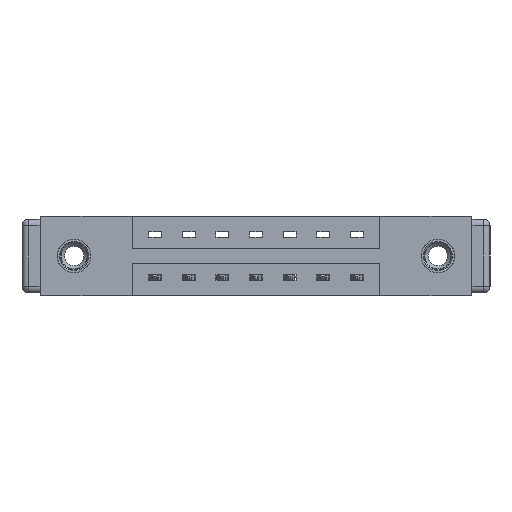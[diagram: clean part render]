
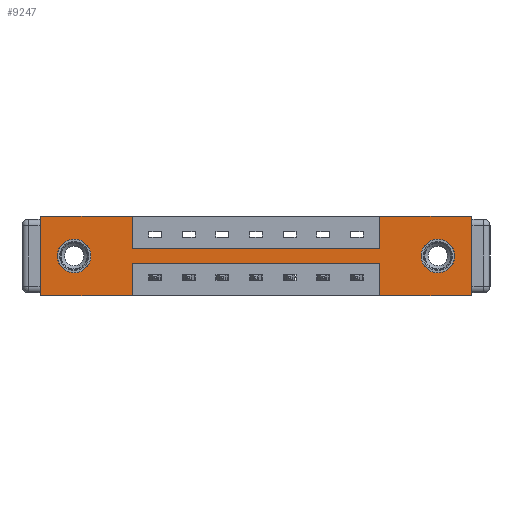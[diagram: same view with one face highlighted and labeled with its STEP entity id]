
A CAD part, front view. The second image highlights one B-rep face of the part: STEP entity #9247.
In plain terms, the highlighted planar face has unit normal (0, -1, 0).
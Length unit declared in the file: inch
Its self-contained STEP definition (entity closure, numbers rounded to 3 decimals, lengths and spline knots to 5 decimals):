
#41 = LINE ( 'NONE', #3227, #10011 ) ;
#83 = EDGE_CURVE ( 'NONE', #3918, #10486, #2257, .T. ) ;
#154 = DIRECTION ( 'NONE',  ( 0., 0., -1. ) ) ;
#155 = EDGE_CURVE ( 'NONE', #5414, #1514, #12267, .T. ) ;
#390 = LINE ( 'NONE', #3840, #11283 ) ;
#429 = AXIS2_PLACEMENT_3D ( 'NONE', #11766, #8809, #8047 ) ;
#773 = VECTOR ( 'NONE', #5761, 39.37008 ) ;
#810 = ORIENTED_EDGE ( 'NONE', *, *, #155, .T. ) ;
#975 = DIRECTION ( 'NONE',  ( 0., 0., 1. ) ) ;
#1060 = CARTESIAN_POINT ( 'NONE',  ( 0.425, 0., -0.22 ) ) ;
#1147 = VECTOR ( 'NONE', #5138, 39.37008 ) ;
#1182 = ORIENTED_EDGE ( 'NONE', *, *, #2270, .T. ) ;
#1375 = LINE ( 'NONE', #10587, #773 ) ;
#1454 = EDGE_CURVE ( 'NONE', #12135, #6594, #2813, .T. ) ;
#1498 = CARTESIAN_POINT ( 'NONE',  ( 0.155, 0., -0.263 ) ) ;
#1514 = VERTEX_POINT ( 'NONE', #2325 ) ;
#1581 = DIRECTION ( 'NONE',  ( 1., 0., 0. ) ) ;
#1786 = VECTOR ( 'NONE', #6313, 39.37008 ) ;
#1788 = CARTESIAN_POINT ( 'NONE',  ( 0.425, 0., -0.37 ) ) ;
#1835 = DIRECTION ( 'NONE',  ( 1., 0., 0. ) ) ;
#1883 = LINE ( 'NONE', #5385, #12038 ) ;
#1897 = VERTEX_POINT ( 'NONE', #5158 ) ;
#2151 = CARTESIAN_POINT ( 'NONE',  ( 0.155, 0., -0.185 ) ) ;
#2257 = LINE ( 'NONE', #3065, #8626 ) ;
#2270 = EDGE_CURVE ( 'NONE', #9743, #3551, #11483, .T. ) ;
#2309 = EDGE_CURVE ( 'NONE', #3551, #9743, #4194, .T. ) ;
#2325 = CARTESIAN_POINT ( 'NONE',  ( 1.843, 0., -0.263 ) ) ;
#2339 = EDGE_LOOP ( 'NONE', ( #3358, #3071, #7086, #3645, #11951, #3665, #6571, #7461, #10893, #12211, #9623, #10466 ) ) ;
#2487 = DIRECTION ( 'NONE',  ( 0., 1., 0. ) ) ;
#2681 = AXIS2_PLACEMENT_3D ( 'NONE', #10922, #7076, #11890 ) ;
#2778 = DIRECTION ( 'NONE',  ( 0., 0., -1. ) ) ;
#2813 = LINE ( 'NONE', #11980, #1786 ) ;
#2863 = CARTESIAN_POINT ( 'NONE',  ( 0., 0., 0. ) ) ;
#2952 = EDGE_CURVE ( 'NONE', #7847, #11902, #11616, .T. ) ;
#3065 = CARTESIAN_POINT ( 'NONE',  ( 0., 0., 0. ) ) ;
#3071 = ORIENTED_EDGE ( 'NONE', *, *, #2952, .F. ) ;
#3073 = DIRECTION ( 'NONE',  ( -1., 0., 0. ) ) ;
#3104 = DIRECTION ( 'NONE',  ( -1., 0., 0. ) ) ;
#3227 = CARTESIAN_POINT ( 'NONE',  ( 1.573, 0., -0.37 ) ) ;
#3345 = AXIS2_PLACEMENT_3D ( 'NONE', #2151, #4499, #4542 ) ;
#3358 = ORIENTED_EDGE ( 'NONE', *, *, #10921, .F. ) ;
#3420 = VERTEX_POINT ( 'NONE', #6747 ) ;
#3512 = LINE ( 'NONE', #2863, #6861 ) ;
#3551 = VERTEX_POINT ( 'NONE', #1498 ) ;
#3641 = LINE ( 'NONE', #1788, #9851 ) ;
#3645 = ORIENTED_EDGE ( 'NONE', *, *, #10880, .F. ) ;
#3658 = CIRCLE ( 'NONE', #6306, 0.078 ) ;
#3665 = ORIENTED_EDGE ( 'NONE', *, *, #9905, .F. ) ;
#3703 = EDGE_CURVE ( 'NONE', #11402, #1897, #1883, .T. ) ;
#3739 = DIRECTION ( 'NONE',  ( 1., 0., 0. ) ) ;
#3840 = CARTESIAN_POINT ( 'NONE',  ( 0., 0., -0.37 ) ) ;
#3856 = VERTEX_POINT ( 'NONE', #5665 ) ;
#3918 = VERTEX_POINT ( 'NONE', #7196 ) ;
#3981 = EDGE_CURVE ( 'NONE', #8940, #11402, #12199, .T. ) ;
#4194 = CIRCLE ( 'NONE', #3345, 0.078 ) ;
#4242 = EDGE_CURVE ( 'NONE', #3856, #3918, #390, .T. ) ;
#4284 = LINE ( 'NONE', #9673, #9581 ) ;
#4499 = DIRECTION ( 'NONE',  ( 0., 1., 0. ) ) ;
#4542 = DIRECTION ( 'NONE',  ( 0., 0., 1. ) ) ;
#4749 = CARTESIAN_POINT ( 'NONE',  ( 1.998, 0., 0. ) ) ;
#4985 = PLANE ( 'NONE',  #429 ) ;
#5138 = DIRECTION ( 'NONE',  ( 0., 0., -1. ) ) ;
#5154 = CARTESIAN_POINT ( 'NONE',  ( 1.998, 0., -0.37 ) ) ;
#5158 = CARTESIAN_POINT ( 'NONE',  ( 1.573, 0., -0.15 ) ) ;
#5220 = ORIENTED_EDGE ( 'NONE', *, *, #6492, .T. ) ;
#5385 = CARTESIAN_POINT ( 'NONE',  ( 0.425, 0., -0.15 ) ) ;
#5414 = VERTEX_POINT ( 'NONE', #11167 ) ;
#5500 = FACE_BOUND ( 'NONE', #11886, .T. ) ;
#5665 = CARTESIAN_POINT ( 'NONE',  ( 0.425, 0., -0.37 ) ) ;
#5761 = DIRECTION ( 'NONE',  ( -1., 0., 0. ) ) ;
#5919 = DIRECTION ( 'NONE',  ( 0., 1., 0. ) ) ;
#6306 = AXIS2_PLACEMENT_3D ( 'NONE', #10741, #5919, #154 ) ;
#6313 = DIRECTION ( 'NONE',  ( 0., 0., -1. ) ) ;
#6492 = EDGE_CURVE ( 'NONE', #1514, #5414, #3658, .T. ) ;
#6521 = LINE ( 'NONE', #10558, #11065 ) ;
#6571 = ORIENTED_EDGE ( 'NONE', *, *, #6641, .F. ) ;
#6579 = VERTEX_POINT ( 'NONE', #7960 ) ;
#6594 = VERTEX_POINT ( 'NONE', #5154 ) ;
#6641 = EDGE_CURVE ( 'NONE', #1897, #6579, #6521, .T. ) ;
#6714 = DIRECTION ( 'NONE',  ( 0., 0., 1. ) ) ;
#6747 = CARTESIAN_POINT ( 'NONE',  ( 1.573, 0., -0.37 ) ) ;
#6828 = EDGE_CURVE ( 'NONE', #3420, #7847, #41, .T. ) ;
#6861 = VECTOR ( 'NONE', #1835, 39.37008 ) ;
#6926 = CARTESIAN_POINT ( 'NONE',  ( 0., 0., 0. ) ) ;
#7076 = DIRECTION ( 'NONE',  ( 0., 1., 0. ) ) ;
#7086 = ORIENTED_EDGE ( 'NONE', *, *, #6828, .F. ) ;
#7110 = EDGE_LOOP ( 'NONE', ( #810, #5220 ) ) ;
#7196 = CARTESIAN_POINT ( 'NONE',  ( 0., 0., -0.37 ) ) ;
#7212 = VECTOR ( 'NONE', #3104, 39.37008 ) ;
#7377 = DIRECTION ( 'NONE',  ( 0., 0., -1. ) ) ;
#7461 = ORIENTED_EDGE ( 'NONE', *, *, #3703, .F. ) ;
#7768 = CARTESIAN_POINT ( 'NONE',  ( 0.425, 0., -0.22 ) ) ;
#7804 = CARTESIAN_POINT ( 'NONE',  ( 1.843, 0., -0.185 ) ) ;
#7847 = VERTEX_POINT ( 'NONE', #9254 ) ;
#7960 = CARTESIAN_POINT ( 'NONE',  ( 1.573, 0., 0. ) ) ;
#8047 = DIRECTION ( 'NONE',  ( 0., 0., -1. ) ) ;
#8166 = DIRECTION ( 'NONE',  ( 0., 0., 1. ) ) ;
#8626 = VECTOR ( 'NONE', #975, 39.37008 ) ;
#8809 = DIRECTION ( 'NONE',  ( 0., -1., 0. ) ) ;
#8819 = CARTESIAN_POINT ( 'NONE',  ( 0.425, 0., 0. ) ) ;
#8940 = VERTEX_POINT ( 'NONE', #8819 ) ;
#9247 = ADVANCED_FACE ( 'NONE', ( #11116, #5500, #9607 ), #4985, .T. ) ;
#9254 = CARTESIAN_POINT ( 'NONE',  ( 1.573, 0., -0.22 ) ) ;
#9581 = VECTOR ( 'NONE', #3739, 39.37008 ) ;
#9590 = AXIS2_PLACEMENT_3D ( 'NONE', #7804, #2487, #7377 ) ;
#9607 = FACE_OUTER_BOUND ( 'NONE', #2339, .T. ) ;
#9623 = ORIENTED_EDGE ( 'NONE', *, *, #83, .F. ) ;
#9633 = ORIENTED_EDGE ( 'NONE', *, *, #2309, .T. ) ;
#9673 = CARTESIAN_POINT ( 'NONE',  ( 0., 0., 0. ) ) ;
#9743 = VERTEX_POINT ( 'NONE', #10850 ) ;
#9851 = VECTOR ( 'NONE', #2778, 39.37008 ) ;
#9884 = EDGE_CURVE ( 'NONE', #10486, #8940, #3512, .T. ) ;
#9905 = EDGE_CURVE ( 'NONE', #6579, #12135, #4284, .T. ) ;
#10011 = VECTOR ( 'NONE', #8166, 39.37008 ) ;
#10190 = CARTESIAN_POINT ( 'NONE',  ( 0.425, 0., -0.15 ) ) ;
#10466 = ORIENTED_EDGE ( 'NONE', *, *, #4242, .F. ) ;
#10486 = VERTEX_POINT ( 'NONE', #6926 ) ;
#10558 = CARTESIAN_POINT ( 'NONE',  ( 1.573, 0., 0. ) ) ;
#10587 = CARTESIAN_POINT ( 'NONE',  ( 0., 0., -0.37 ) ) ;
#10741 = CARTESIAN_POINT ( 'NONE',  ( 1.843, 0., -0.185 ) ) ;
#10850 = CARTESIAN_POINT ( 'NONE',  ( 0.155, 0., -0.107 ) ) ;
#10880 = EDGE_CURVE ( 'NONE', #6594, #3420, #1375, .T. ) ;
#10893 = ORIENTED_EDGE ( 'NONE', *, *, #3981, .F. ) ;
#10921 = EDGE_CURVE ( 'NONE', #11902, #3856, #3641, .T. ) ;
#10922 = CARTESIAN_POINT ( 'NONE',  ( 0.155, 0., -0.185 ) ) ;
#10987 = CARTESIAN_POINT ( 'NONE',  ( 0.425, 0., 0. ) ) ;
#11065 = VECTOR ( 'NONE', #6714, 39.37008 ) ;
#11116 = FACE_BOUND ( 'NONE', #7110, .T. ) ;
#11167 = CARTESIAN_POINT ( 'NONE',  ( 1.843, 0., -0.107 ) ) ;
#11283 = VECTOR ( 'NONE', #3073, 39.37008 ) ;
#11402 = VERTEX_POINT ( 'NONE', #10190 ) ;
#11483 = CIRCLE ( 'NONE', #2681, 0.078 ) ;
#11616 = LINE ( 'NONE', #1060, #7212 ) ;
#11766 = CARTESIAN_POINT ( 'NONE',  ( 0., 0., -0.37 ) ) ;
#11886 = EDGE_LOOP ( 'NONE', ( #1182, #9633 ) ) ;
#11890 = DIRECTION ( 'NONE',  ( 0., 0., 1. ) ) ;
#11902 = VERTEX_POINT ( 'NONE', #7768 ) ;
#11951 = ORIENTED_EDGE ( 'NONE', *, *, #1454, .F. ) ;
#11980 = CARTESIAN_POINT ( 'NONE',  ( 1.998, 0., 0. ) ) ;
#12038 = VECTOR ( 'NONE', #1581, 39.37008 ) ;
#12135 = VERTEX_POINT ( 'NONE', #4749 ) ;
#12199 = LINE ( 'NONE', #10987, #1147 ) ;
#12211 = ORIENTED_EDGE ( 'NONE', *, *, #9884, .F. ) ;
#12267 = CIRCLE ( 'NONE', #9590, 0.078 ) ;
